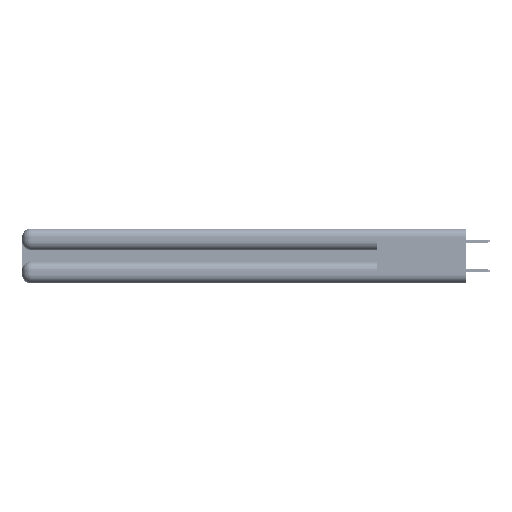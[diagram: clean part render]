
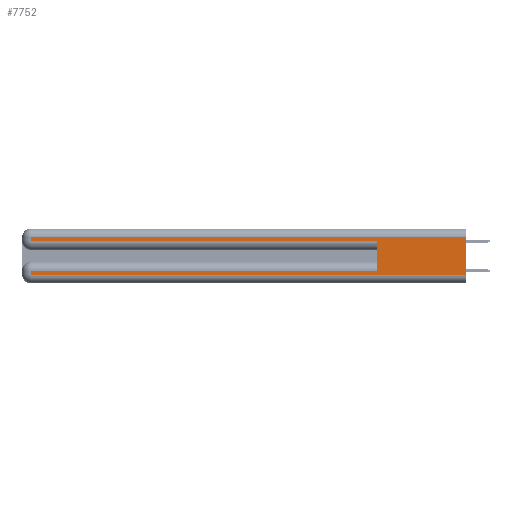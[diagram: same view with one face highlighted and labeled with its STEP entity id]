
A CAD part, left-side view. The second image highlights one B-rep face of the part: STEP entity #7752.
In plain terms, the highlighted planar face has unit normal (-1, 0, 0).
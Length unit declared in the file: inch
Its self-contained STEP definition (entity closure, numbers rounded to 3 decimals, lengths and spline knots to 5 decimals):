
#879 = ORIENTED_EDGE ( 'NONE', *, *, #9197, .F. ) ;
#3412 = LINE ( 'NONE', #6009, #13792 ) ;
#4347 = AXIS2_PLACEMENT_3D ( 'NONE', #20344, #33872, #33478 ) ;
#4665 = LINE ( 'NONE', #5596, #6769 ) ;
#4771 = CARTESIAN_POINT ( 'NONE',  ( 0., 0., 0.085 ) ) ;
#4777 = CARTESIAN_POINT ( 'NONE',  ( 0., 2.94, 0.37 ) ) ;
#4837 = VERTEX_POINT ( 'NONE', #57101 ) ;
#5596 = CARTESIAN_POINT ( 'NONE',  ( 0., 0., 0.285 ) ) ;
#5895 = CARTESIAN_POINT ( 'NONE',  ( 0., 2.94, 0.285 ) ) ;
#6009 = CARTESIAN_POINT ( 'NONE',  ( 0., 0., 0.31 ) ) ;
#6169 = EDGE_CURVE ( 'NONE', #24272, #26806, #44965, .T. ) ;
#6613 = CARTESIAN_POINT ( 'NONE',  ( 0., 2.94, 0.37 ) ) ;
#6769 = VECTOR ( 'NONE', #54545, 39.37008 ) ;
#7752 = ADVANCED_FACE ( 'NONE', ( #44074 ), #33283, .F. ) ;
#8624 = DIRECTION ( 'NONE',  ( 0., 0., -1. ) ) ;
#9002 = CARTESIAN_POINT ( 'NONE',  ( 0., 0.6, 0.085 ) ) ;
#9197 = EDGE_CURVE ( 'NONE', #40711, #15941, #46725, .T. ) ;
#9472 = ORIENTED_EDGE ( 'NONE', *, *, #6169, .T. ) ;
#10352 = CARTESIAN_POINT ( 'NONE',  ( 0., 0., 0.31 ) ) ;
#10633 = EDGE_CURVE ( 'NONE', #26806, #4837, #4665, .T. ) ;
#13273 = DIRECTION ( 'NONE',  ( 0., 0., -1. ) ) ;
#13792 = VECTOR ( 'NONE', #54946, 39.37008 ) ;
#15941 = VERTEX_POINT ( 'NONE', #41015 ) ;
#17178 = EDGE_CURVE ( 'NONE', #24004, #15941, #29525, .T. ) ;
#17924 = EDGE_LOOP ( 'NONE', ( #879, #51770, #9472, #32756, #30976, #38149, #23110, #46649 ) ) ;
#17934 = VECTOR ( 'NONE', #53505, 39.37008 ) ;
#19518 = EDGE_CURVE ( 'NONE', #40711, #24272, #3412, .T. ) ;
#19668 = CARTESIAN_POINT ( 'NONE',  ( 0., 2.94, 0.085 ) ) ;
#19722 = CARTESIAN_POINT ( 'NONE',  ( 0., 2.94, 0.06 ) ) ;
#20344 = CARTESIAN_POINT ( 'NONE',  ( 0., 0., 0.37 ) ) ;
#20901 = DIRECTION ( 'NONE',  ( 0., 0., 1. ) ) ;
#21164 = VERTEX_POINT ( 'NONE', #9002 ) ;
#23110 = ORIENTED_EDGE ( 'NONE', *, *, #38096, .T. ) ;
#23507 = DIRECTION ( 'NONE',  ( 0., -1., 0. ) ) ;
#24004 = VERTEX_POINT ( 'NONE', #19722 ) ;
#24272 = VERTEX_POINT ( 'NONE', #42940 ) ;
#24975 = LINE ( 'NONE', #55885, #33406 ) ;
#26806 = VERTEX_POINT ( 'NONE', #5895 ) ;
#28784 = VECTOR ( 'NONE', #38762, 39.37008 ) ;
#29525 = LINE ( 'NONE', #37180, #43423 ) ;
#30877 = LINE ( 'NONE', #6613, #28784 ) ;
#30976 = ORIENTED_EDGE ( 'NONE', *, *, #34597, .F. ) ;
#32756 = ORIENTED_EDGE ( 'NONE', *, *, #10633, .T. ) ;
#33218 = VERTEX_POINT ( 'NONE', #19668 ) ;
#33283 = PLANE ( 'NONE',  #4347 ) ;
#33406 = VECTOR ( 'NONE', #20901, 39.37008 ) ;
#33478 = DIRECTION ( 'NONE',  ( 0., 0., -1. ) ) ;
#33872 = DIRECTION ( 'NONE',  ( 1., 0., 0. ) ) ;
#34597 = EDGE_CURVE ( 'NONE', #21164, #4837, #24975, .T. ) ;
#34771 = EDGE_CURVE ( 'NONE', #21164, #33218, #52194, .T. ) ;
#37180 = CARTESIAN_POINT ( 'NONE',  ( 0., 0., 0.06 ) ) ;
#38096 = EDGE_CURVE ( 'NONE', #33218, #24004, #30877, .T. ) ;
#38149 = ORIENTED_EDGE ( 'NONE', *, *, #34771, .T. ) ;
#38762 = DIRECTION ( 'NONE',  ( 0., 0., -1. ) ) ;
#40711 = VERTEX_POINT ( 'NONE', #10352 ) ;
#41015 = CARTESIAN_POINT ( 'NONE',  ( 0., 0., 0.06 ) ) ;
#42940 = CARTESIAN_POINT ( 'NONE',  ( 0., 2.94, 0.31 ) ) ;
#43423 = VECTOR ( 'NONE', #23507, 39.37008 ) ;
#44074 = FACE_OUTER_BOUND ( 'NONE', #17924, .T. ) ;
#44902 = VECTOR ( 'NONE', #13273, 39.37008 ) ;
#44965 = LINE ( 'NONE', #4777, #44902 ) ;
#46649 = ORIENTED_EDGE ( 'NONE', *, *, #17178, .T. ) ;
#46725 = LINE ( 'NONE', #57228, #54429 ) ;
#51770 = ORIENTED_EDGE ( 'NONE', *, *, #19518, .T. ) ;
#52194 = LINE ( 'NONE', #4771, #17934 ) ;
#53505 = DIRECTION ( 'NONE',  ( 0., 1., 0. ) ) ;
#54429 = VECTOR ( 'NONE', #8624, 39.37008 ) ;
#54545 = DIRECTION ( 'NONE',  ( 0., -1., 0. ) ) ;
#54946 = DIRECTION ( 'NONE',  ( 0., 1., 0. ) ) ;
#55885 = CARTESIAN_POINT ( 'NONE',  ( 0., 0.6, 0.145 ) ) ;
#57101 = CARTESIAN_POINT ( 'NONE',  ( 0., 0.6, 0.285 ) ) ;
#57228 = CARTESIAN_POINT ( 'NONE',  ( 0., 0., 0.37 ) ) ;
